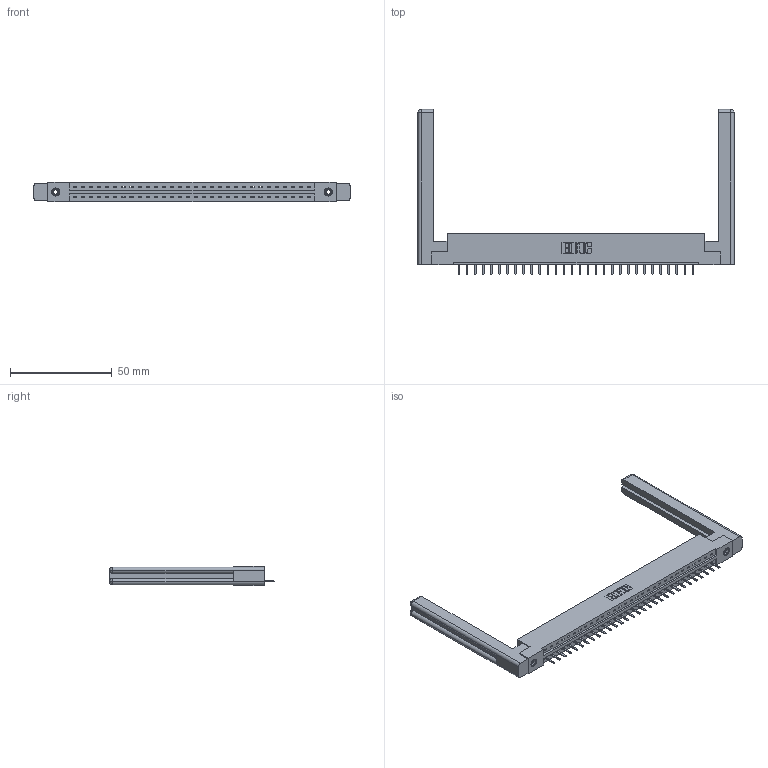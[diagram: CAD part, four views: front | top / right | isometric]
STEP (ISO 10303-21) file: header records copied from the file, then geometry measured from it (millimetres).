
FILE_DESCRIPTION (( 'STEP AP203' ), '1' );
FILE_NAME ('387-030-520-158.STEP', '2019-10-03T17:43:25', ( '' ), ( '' ), 'SwSTEP 2.0', 'SolidWorks 2016', '' );
FILE_SCHEMA (( 'CONFIG_CONTROL_DESIGN' ));
Length unit declared in the file: inch
Products named in the file (5): 345-250-001_345-250-001-102; 345-292-001_345-293-120; 307-220-058; 387-030-520-158; 337 Part_Flush Mounting Lugs - 0.156 Dia-TI
Assembly tree (35 placements, depth 2):
  387-030-520-158
    337 Part_Flush Mounting Lugs - 0.156 Dia-TI
    345-292-001_345-293-120  x30
    345-250-001_345-250-001-102  x2
    307-220-058  x2
Bounding box: 155.5 x 81.11 x 9.4 mm (x, y, z)
Volume: 23087.2 mm3; surface area: 21292 mm2
Topology: 35 solids, 35 shells, 2236 faces, 6545 edges, 4270 vertices
Faces by surface type: plane 1594, cylinder 618, cone 12, torus 12
Entity records: 26600 total; most frequent: CARTESIAN_POINT 4643, ORIENTED_EDGE 4536, DIRECTION 3940, EDGE_CURVE 2268, LINE 2088, VECTOR 2088, VERTEX_POINT 1502, AXIS2_PLACEMENT_3D 926
